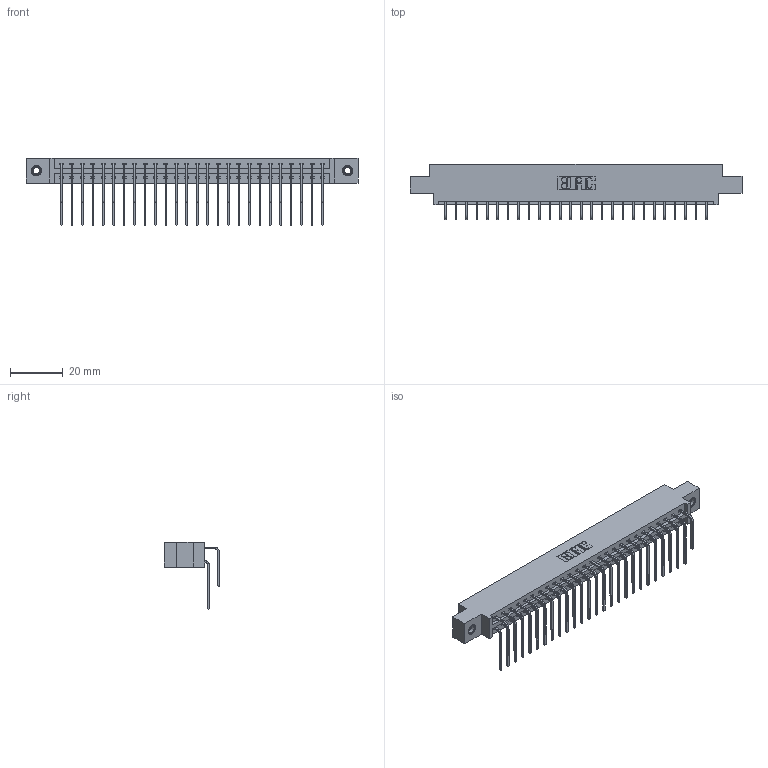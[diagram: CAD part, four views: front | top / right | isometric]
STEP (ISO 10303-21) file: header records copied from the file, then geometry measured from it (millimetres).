
FILE_DESCRIPTION (( 'STEP AP203' ), '1' );
FILE_NAME ('337-052-559-807.STEP', '2018-08-09T23:44:45', ( '' ), ( '' ), 'SwSTEP 2.0', 'SolidWorks 2016', '' );
FILE_SCHEMA (( 'CONFIG_CONTROL_DESIGN' ));
Length unit declared in the file: inch
Products named in the file (5): 345-250-001_345-250-005-103; 337-052-559-807; 337 Part_0.170 Offset - 0.156 Dia-TI; 345-292-001_558 559 Tail - 1; 345-292-001_559 Tail - 2
Assembly tree (55 placements, depth 2):
  337-052-559-807
    337 Part_0.170 Offset - 0.156 Dia-TI
    345-292-001_558 559 Tail - 1  x26
    345-292-001_559 Tail - 2  x26
    345-250-001_345-250-005-103  x2
Bounding box: 126.03 x 20.9 x 25.53 mm (x, y, z)
Volume: 13238.5 mm3; surface area: 16460.8 mm2
Topology: 55 solids, 55 shells, 3090 faces, 9143 edges, 6018 vertices
Faces by surface type: plane 2186, cylinder 888, cone 12, torus 4
Entity records: 25330 total; most frequent: CARTESIAN_POINT 4308, ORIENTED_EDGE 4186, DIRECTION 3707, EDGE_CURVE 2093, VECTOR 1905, LINE 1905, VERTEX_POINT 1388, AXIS2_PLACEMENT_3D 901
